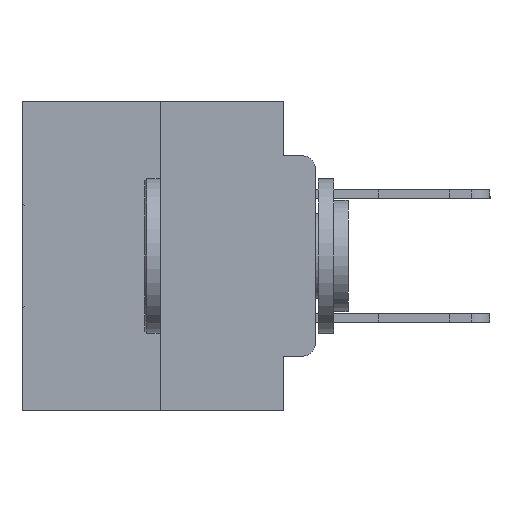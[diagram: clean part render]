
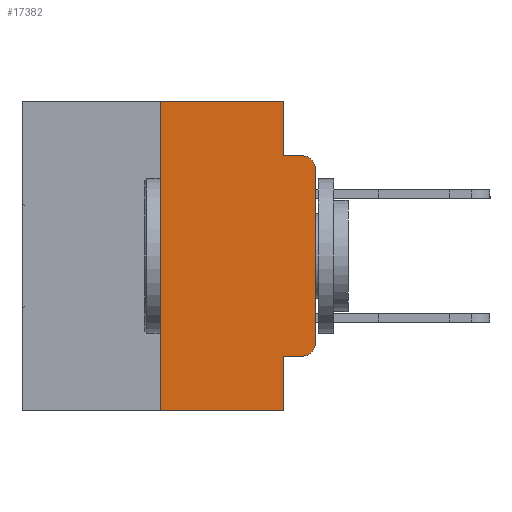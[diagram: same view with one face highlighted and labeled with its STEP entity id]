
A CAD part, left-side view. The second image highlights one B-rep face of the part: STEP entity #17382.
In plain terms, the highlighted planar face has unit normal (-1, 0, 0).
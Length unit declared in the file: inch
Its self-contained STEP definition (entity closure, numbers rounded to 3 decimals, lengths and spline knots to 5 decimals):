
#266 = EDGE_CURVE ( 'NONE', #9861, #27575, #25628, .T. ) ;
#606 = VECTOR ( 'NONE', #16243, 39.37008 ) ;
#684 = AXIS2_PLACEMENT_3D ( 'NONE', #23618, #23775, #19502 ) ;
#742 = ORIENTED_EDGE ( 'NONE', *, *, #266, .F. ) ;
#1860 = ORIENTED_EDGE ( 'NONE', *, *, #8176, .T. ) ;
#2218 = EDGE_CURVE ( 'NONE', #30301, #28554, #16706, .T. ) ;
#2324 = VECTOR ( 'NONE', #18712, 39.37008 ) ;
#2482 = EDGE_LOOP ( 'NONE', ( #8379, #9525, #742, #12155, #24677, #19893, #1860, #21400, #10313, #29027 ) ) ;
#3080 = EDGE_CURVE ( 'NONE', #24420, #8887, #23637, .T. ) ;
#3097 = LINE ( 'NONE', #28135, #2324 ) ;
#3445 = CARTESIAN_POINT ( 'NONE',  ( 0., 0.02, -0.1085 ) ) ;
#3563 = FACE_OUTER_BOUND ( 'NONE', #2482, .T. ) ;
#4160 = CARTESIAN_POINT ( 'NONE',  ( 0., 0.051, -0.4115 ) ) ;
#4545 = LINE ( 'NONE', #9212, #10014 ) ;
#4699 = CARTESIAN_POINT ( 'NONE',  ( 0., 0., -0.1085 ) ) ;
#5315 = VECTOR ( 'NONE', #21676, 39.37008 ) ;
#5773 = DIRECTION ( 'NONE',  ( 0., 0., -1. ) ) ;
#7113 = CARTESIAN_POINT ( 'NONE',  ( 0., 0.25, -0.5 ) ) ;
#8176 = EDGE_CURVE ( 'NONE', #13210, #8887, #18521, .T. ) ;
#8379 = ORIENTED_EDGE ( 'NONE', *, *, #29910, .T. ) ;
#8656 = VECTOR ( 'NONE', #8914, 39.37008 ) ;
#8716 = EDGE_CURVE ( 'NONE', #13210, #28283, #3097, .T. ) ;
#8814 = VECTOR ( 'NONE', #27662, 39.37008 ) ;
#8887 = VERTEX_POINT ( 'NONE', #12327 ) ;
#8914 = DIRECTION ( 'NONE',  ( 0., -1., 0. ) ) ;
#9132 = CIRCLE ( 'NONE', #9165, 0.02 ) ;
#9165 = AXIS2_PLACEMENT_3D ( 'NONE', #3445, #19853, #5773 ) ;
#9212 = CARTESIAN_POINT ( 'NONE',  ( 0., 0., 0. ) ) ;
#9525 = ORIENTED_EDGE ( 'NONE', *, *, #14489, .T. ) ;
#9538 = VERTEX_POINT ( 'NONE', #26485 ) ;
#9551 = LINE ( 'NONE', #4160, #8814 ) ;
#9607 = AXIS2_PLACEMENT_3D ( 'NONE', #22281, #29247, #15257 ) ;
#9861 = VERTEX_POINT ( 'NONE', #18240 ) ;
#9876 = EDGE_CURVE ( 'NONE', #24420, #30301, #9551, .T. ) ;
#10014 = VECTOR ( 'NONE', #21010, 39.37008 ) ;
#10313 = ORIENTED_EDGE ( 'NONE', *, *, #9876, .T. ) ;
#10339 = LINE ( 'NONE', #21966, #21430 ) ;
#12155 = ORIENTED_EDGE ( 'NONE', *, *, #19787, .F. ) ;
#12327 = CARTESIAN_POINT ( 'NONE',  ( 0., 0.051, -0.5 ) ) ;
#12872 = PLANE ( 'NONE',  #9607 ) ;
#13210 = VERTEX_POINT ( 'NONE', #7113 ) ;
#14489 = EDGE_CURVE ( 'NONE', #28864, #27575, #9132, .T. ) ;
#14835 = CARTESIAN_POINT ( 'NONE',  ( 0., 0., -0.3915 ) ) ;
#15257 = DIRECTION ( 'NONE',  ( 0., 0., -1. ) ) ;
#15917 = CARTESIAN_POINT ( 'NONE',  ( 0., 0.051, -0.0885 ) ) ;
#16243 = DIRECTION ( 'NONE',  ( 0., -1., 0. ) ) ;
#16706 = CIRCLE ( 'NONE', #684, 0.02 ) ;
#17382 = ADVANCED_FACE ( 'NONE', ( #3563 ), #12872, .F. ) ;
#17586 = CARTESIAN_POINT ( 'NONE',  ( 0., 0.051, -0.4115 ) ) ;
#18240 = CARTESIAN_POINT ( 'NONE',  ( 0., 0.051, -0.0885 ) ) ;
#18521 = LINE ( 'NONE', #28565, #5315 ) ;
#18712 = DIRECTION ( 'NONE',  ( 0., 0., 1. ) ) ;
#19502 = DIRECTION ( 'NONE',  ( 0., 0., -1. ) ) ;
#19787 = EDGE_CURVE ( 'NONE', #9538, #9861, #10339, .T. ) ;
#19853 = DIRECTION ( 'NONE',  ( -1., 0., 0. ) ) ;
#19893 = ORIENTED_EDGE ( 'NONE', *, *, #8716, .F. ) ;
#20130 = CARTESIAN_POINT ( 'NONE',  ( 0., 0.02, -0.4115 ) ) ;
#20275 = DIRECTION ( 'NONE',  ( 0., 0., -1. ) ) ;
#21010 = DIRECTION ( 'NONE',  ( 0., 0., 1. ) ) ;
#21400 = ORIENTED_EDGE ( 'NONE', *, *, #3080, .F. ) ;
#21430 = VECTOR ( 'NONE', #24270, 39.37008 ) ;
#21676 = DIRECTION ( 'NONE',  ( 0., -1., 0. ) ) ;
#21966 = CARTESIAN_POINT ( 'NONE',  ( 0., 0.051, 0. ) ) ;
#22281 = CARTESIAN_POINT ( 'NONE',  ( 0., 0.473, 0. ) ) ;
#23055 = CARTESIAN_POINT ( 'NONE',  ( 0., 0.473, 0. ) ) ;
#23618 = CARTESIAN_POINT ( 'NONE',  ( 0., 0.02, -0.3915 ) ) ;
#23637 = LINE ( 'NONE', #26564, #29755 ) ;
#23775 = DIRECTION ( 'NONE',  ( -1., 0., 0. ) ) ;
#24270 = DIRECTION ( 'NONE',  ( 0., 0., -1. ) ) ;
#24420 = VERTEX_POINT ( 'NONE', #17586 ) ;
#24677 = ORIENTED_EDGE ( 'NONE', *, *, #26942, .F. ) ;
#25365 = CARTESIAN_POINT ( 'NONE',  ( 0., 0.02, -0.0885 ) ) ;
#25628 = LINE ( 'NONE', #15917, #606 ) ;
#26485 = CARTESIAN_POINT ( 'NONE',  ( 0., 0.051, 0. ) ) ;
#26564 = CARTESIAN_POINT ( 'NONE',  ( 0., 0.051, 0. ) ) ;
#26942 = EDGE_CURVE ( 'NONE', #28283, #9538, #27433, .T. ) ;
#27433 = LINE ( 'NONE', #23055, #8656 ) ;
#27575 = VERTEX_POINT ( 'NONE', #25365 ) ;
#27662 = DIRECTION ( 'NONE',  ( 0., -1., 0. ) ) ;
#28135 = CARTESIAN_POINT ( 'NONE',  ( 0., 0.25, 0. ) ) ;
#28283 = VERTEX_POINT ( 'NONE', #30104 ) ;
#28554 = VERTEX_POINT ( 'NONE', #14835 ) ;
#28565 = CARTESIAN_POINT ( 'NONE',  ( 0., 0.473, -0.5 ) ) ;
#28864 = VERTEX_POINT ( 'NONE', #4699 ) ;
#29027 = ORIENTED_EDGE ( 'NONE', *, *, #2218, .T. ) ;
#29247 = DIRECTION ( 'NONE',  ( 1., 0., 0. ) ) ;
#29755 = VECTOR ( 'NONE', #20275, 39.37008 ) ;
#29910 = EDGE_CURVE ( 'NONE', #28554, #28864, #4545, .T. ) ;
#30104 = CARTESIAN_POINT ( 'NONE',  ( 0., 0.25, 0. ) ) ;
#30301 = VERTEX_POINT ( 'NONE', #20130 ) ;
